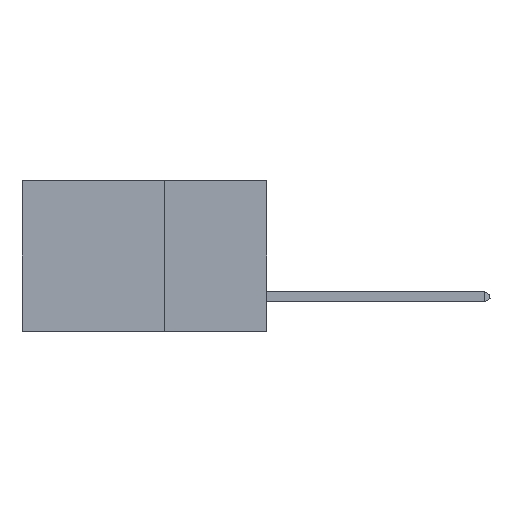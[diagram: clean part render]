
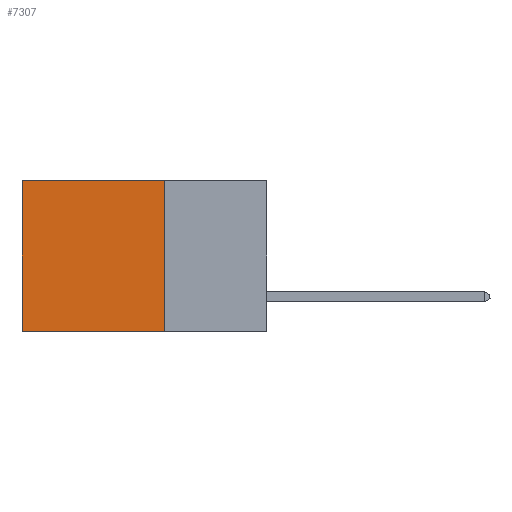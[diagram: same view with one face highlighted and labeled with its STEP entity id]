
A CAD part, left-side view. The second image highlights one B-rep face of the part: STEP entity #7307.
In plain terms, the highlighted planar face has unit normal (-1, 0, 0).
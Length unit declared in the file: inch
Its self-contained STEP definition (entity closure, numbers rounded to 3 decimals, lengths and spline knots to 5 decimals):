
#1184 = CARTESIAN_POINT ( 'NONE',  ( 0.2875, 0.25, 0. ) ) ;
#1449 = ORIENTED_EDGE ( 'NONE', *, *, #11472, .T. ) ;
#2365 = VERTEX_POINT ( 'NONE', #12323 ) ;
#2381 = LINE ( 'NONE', #6952, #11787 ) ;
#2881 = VECTOR ( 'NONE', #11264, 39.37008 ) ;
#3497 = VERTEX_POINT ( 'NONE', #8442 ) ;
#4006 = LINE ( 'NONE', #4450, #8412 ) ;
#4292 = EDGE_LOOP ( 'NONE', ( #1449, #7573, #10932, #11947 ) ) ;
#4416 = FACE_OUTER_BOUND ( 'NONE', #4292, .T. ) ;
#4450 = CARTESIAN_POINT ( 'NONE',  ( 0.2875, 0.25, 0. ) ) ;
#4476 = CARTESIAN_POINT ( 'NONE',  ( 0.2875, 0.25, 0. ) ) ;
#4636 = VERTEX_POINT ( 'NONE', #7687 ) ;
#5101 = AXIS2_PLACEMENT_3D ( 'NONE', #7710, #7662, #9709 ) ;
#5353 = EDGE_CURVE ( 'NONE', #7794, #4636, #4006, .T. ) ;
#6238 = EDGE_CURVE ( 'NONE', #7794, #3497, #9663, .T. ) ;
#6913 = VECTOR ( 'NONE', #9424, 39.37008 ) ;
#6952 = CARTESIAN_POINT ( 'NONE',  ( 0.2875, 0.25, -0.37 ) ) ;
#7307 = ADVANCED_FACE ( 'NONE', ( #4416 ), #10840, .F. ) ;
#7573 = ORIENTED_EDGE ( 'NONE', *, *, #8218, .F. ) ;
#7662 = DIRECTION ( 'NONE',  ( 1., 0., 0. ) ) ;
#7687 = CARTESIAN_POINT ( 'NONE',  ( 0.2875, 0.25, -0.37 ) ) ;
#7710 = CARTESIAN_POINT ( 'NONE',  ( 0.2875, 0.25, 0. ) ) ;
#7794 = VERTEX_POINT ( 'NONE', #4476 ) ;
#8218 = EDGE_CURVE ( 'NONE', #4636, #2365, #2381, .T. ) ;
#8412 = VECTOR ( 'NONE', #8458, 39.37008 ) ;
#8442 = CARTESIAN_POINT ( 'NONE',  ( 0.2875, 0.6, 0. ) ) ;
#8458 = DIRECTION ( 'NONE',  ( 0., 0., -1. ) ) ;
#8578 = CARTESIAN_POINT ( 'NONE',  ( 0.2875, 0.6, 0. ) ) ;
#9424 = DIRECTION ( 'NONE',  ( 0., 0., -1. ) ) ;
#9663 = LINE ( 'NONE', #1184, #2881 ) ;
#9709 = DIRECTION ( 'NONE',  ( 0., 0., -1. ) ) ;
#10840 = PLANE ( 'NONE',  #5101 ) ;
#10932 = ORIENTED_EDGE ( 'NONE', *, *, #5353, .F. ) ;
#10963 = DIRECTION ( 'NONE',  ( 0., 1., 0. ) ) ;
#11264 = DIRECTION ( 'NONE',  ( 0., 1., 0. ) ) ;
#11472 = EDGE_CURVE ( 'NONE', #3497, #2365, #12907, .T. ) ;
#11787 = VECTOR ( 'NONE', #10963, 39.37008 ) ;
#11947 = ORIENTED_EDGE ( 'NONE', *, *, #6238, .T. ) ;
#12323 = CARTESIAN_POINT ( 'NONE',  ( 0.2875, 0.6, -0.37 ) ) ;
#12907 = LINE ( 'NONE', #8578, #6913 ) ;
